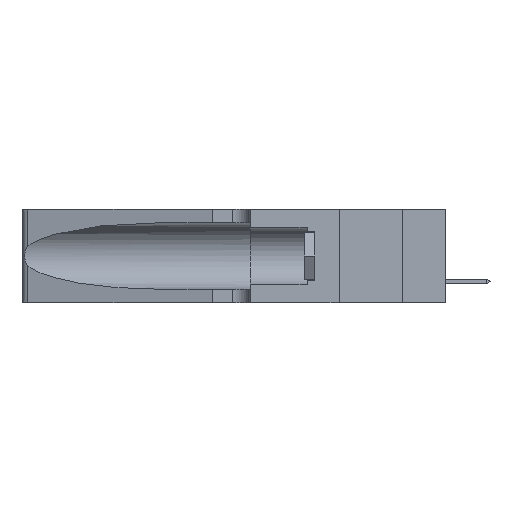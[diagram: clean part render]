
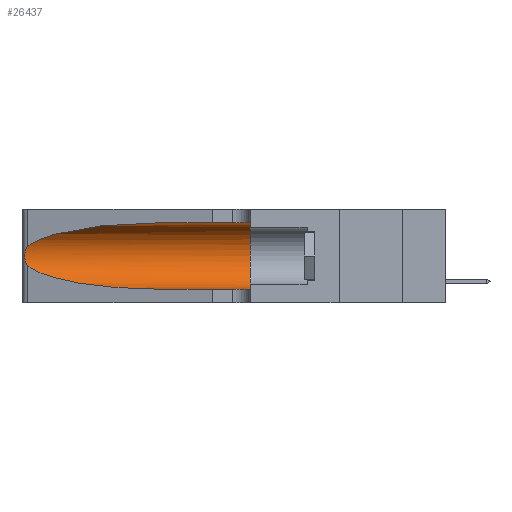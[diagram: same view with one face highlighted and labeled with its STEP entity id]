
A CAD part, left-side view. The second image highlights one B-rep face of the part: STEP entity #26437.
In plain terms, the highlighted cylindrical face has radius 3.308 mm (diameter 6.617 mm), a partial arc.
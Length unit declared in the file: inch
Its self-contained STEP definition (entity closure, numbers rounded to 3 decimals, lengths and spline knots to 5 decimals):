
#262 = CARTESIAN_POINT ( 'NONE',  ( 0.25487, 1.22718, 0.22369 ) ) ;
#280 = AXIS2_PLACEMENT_3D ( 'NONE', #3395, #15954, #1688 ) ;
#473 = CARTESIAN_POINT ( 'NONE',  ( 0.18966, 0.96281, 0.05475 ) ) ;
#739 = ORIENTED_EDGE ( 'NONE', *, *, #21418, .T. ) ;
#1464 = FACE_OUTER_BOUND ( 'NONE', #4771, .T. ) ;
#1688 = DIRECTION ( 'NONE',  ( 0., 0., 1. ) ) ;
#2422 = VECTOR ( 'NONE', #12850, 39.37008 ) ;
#2750 = CARTESIAN_POINT ( 'NONE',  ( 0.1305, 0.72297, 0.05475 ) ) ;
#2774 = CYLINDRICAL_SURFACE ( 'NONE', #20808, 0.13025 ) ;
#3172 = EDGE_CURVE ( 'NONE', #17405, #14031, #8732, .T. ) ;
#3395 = CARTESIAN_POINT ( 'NONE',  ( 0.1305, 0.35, 0.185 ) ) ;
#3426 =( BOUNDED_CURVE ( )  B_SPLINE_CURVE ( 3, ( #11892, #24066, #5710, #11695 ),
 .UNSPECIFIED., .F., .F. ) 
 B_SPLINE_CURVE_WITH_KNOTS ( ( 4, 4 ),
 ( 1.5708, 2.84003 ),
 .UNSPECIFIED. ) 
 CURVE ( )  GEOMETRIC_REPRESENTATION_ITEM ( )  RATIONAL_B_SPLINE_CURVE ( ( 1., 0.87, 0.87, 1. ) ) 
 REPRESENTATION_ITEM ( '' )  );
#4771 = EDGE_LOOP ( 'NONE', ( #6231, #12596, #739, #5840, #10769, #9035 ) ) ;
#5710 = CARTESIAN_POINT ( 'NONE',  ( 0.2373, 1.15595, 0.28018 ) ) ;
#5840 = ORIENTED_EDGE ( 'NONE', *, *, #8519, .T. ) ;
#5871 = CARTESIAN_POINT ( 'NONE',  ( 0.26075, 1.23896, 0.19203 ) ) ;
#6231 = ORIENTED_EDGE ( 'NONE', *, *, #8650, .T. ) ;
#6250 = CARTESIAN_POINT ( 'NONE',  ( 0.1305, 1.61858, 0.185 ) ) ;
#6692 = B_SPLINE_CURVE_WITH_KNOTS ( 'NONE', 3,
 ( #9997, #18161, #20067, #20337, #9913, #26435, #5871, #24551, #7944, #8099, #17982, #26612, #24391, #8023 ),
 .UNSPECIFIED., .F., .F.,
 ( 4, 2, 2, 2, 2, 2, 4 ),
 ( 0., 0.00027, 0.00053, 0.00107, 0.0016, 0.00187, 0.00214 ),
 .UNSPECIFIED. ) ;
#7007 = CARTESIAN_POINT ( 'NONE',  ( 0.25487, 1.22718, 0.14631 ) ) ;
#7218 = CARTESIAN_POINT ( 'NONE',  ( 0.1305, 0.35, 0.31525 ) ) ;
#7944 = CARTESIAN_POINT ( 'NONE',  ( 0.26017, 1.23833, 0.17102 ) ) ;
#8023 = CARTESIAN_POINT ( 'NONE',  ( 0.25487, 1.22718, 0.14631 ) ) ;
#8099 = CARTESIAN_POINT ( 'NONE',  ( 0.25856, 1.23593, 0.16098 ) ) ;
#8519 = EDGE_CURVE ( 'NONE', #26470, #14031, #17799, .T. ) ;
#8650 = EDGE_CURVE ( 'NONE', #16232, #22235, #3426, .T. ) ;
#8732 = CIRCLE ( 'NONE', #280, 0.13025 ) ;
#9035 = ORIENTED_EDGE ( 'NONE', *, *, #17754, .F. ) ;
#9550 = CARTESIAN_POINT ( 'NONE',  ( 0.1305, 0.35, 0.05475 ) ) ;
#9913 = CARTESIAN_POINT ( 'NONE',  ( 0.25854, 1.2359, 0.20912 ) ) ;
#9997 = CARTESIAN_POINT ( 'NONE',  ( 0.25487, 1.22718, 0.22369 ) ) ;
#10358 = CARTESIAN_POINT ( 'NONE',  ( 0.1305, 0.72297, 0.05475 ) ) ;
#10769 = ORIENTED_EDGE ( 'NONE', *, *, #3172, .F. ) ;
#11212 = EDGE_CURVE ( 'NONE', #22235, #25212, #6692, .T. ) ;
#11695 = CARTESIAN_POINT ( 'NONE',  ( 0.25487, 1.22718, 0.22369 ) ) ;
#11892 = CARTESIAN_POINT ( 'NONE',  ( 0.1305, 0.72297, 0.31525 ) ) ;
#12054 = VECTOR ( 'NONE', #23234, 39.37008 ) ;
#12596 = ORIENTED_EDGE ( 'NONE', *, *, #11212, .T. ) ;
#12850 = DIRECTION ( 'NONE',  ( 0., -1., 0. ) ) ;
#13142 = CARTESIAN_POINT ( 'NONE',  ( 0.1305, 1.61858, 0.05475 ) ) ;
#14031 = VERTEX_POINT ( 'NONE', #9550 ) ;
#14220 = CARTESIAN_POINT ( 'NONE',  ( 0.1305, 0.72297, 0.31525 ) ) ;
#14413 = DIRECTION ( 'NONE',  ( 0., -1., 0. ) ) ;
#14416 = CARTESIAN_POINT ( 'NONE',  ( 0.2373, 1.15595, 0.08982 ) ) ;
#15954 = DIRECTION ( 'NONE',  ( 0., 1., 0. ) ) ;
#16232 = VERTEX_POINT ( 'NONE', #14220 ) ;
#16813 = CARTESIAN_POINT ( 'NONE',  ( 0.1305, 1.61858, 0.31525 ) ) ;
#17049 =( BOUNDED_CURVE ( )  B_SPLINE_CURVE ( 3, ( #22644, #14416, #473, #2750 ),
 .UNSPECIFIED., .F., .F. ) 
 B_SPLINE_CURVE_WITH_KNOTS ( ( 4, 4 ),
 ( 3.44316, 4.71239 ),
 .UNSPECIFIED. ) 
 CURVE ( )  GEOMETRIC_REPRESENTATION_ITEM ( )  RATIONAL_B_SPLINE_CURVE ( ( 1., 0.87, 0.87, 1. ) ) 
 REPRESENTATION_ITEM ( '' )  );
#17405 = VERTEX_POINT ( 'NONE', #7218 ) ;
#17754 = EDGE_CURVE ( 'NONE', #16232, #17405, #19443, .T. ) ;
#17799 = LINE ( 'NONE', #13142, #12054 ) ;
#17982 = CARTESIAN_POINT ( 'NONE',  ( 0.25789, 1.23486, 0.15765 ) ) ;
#18161 = CARTESIAN_POINT ( 'NONE',  ( 0.25555, 1.22994, 0.2215 ) ) ;
#19443 = LINE ( 'NONE', #16813, #2422 ) ;
#20067 = CARTESIAN_POINT ( 'NONE',  ( 0.25639, 1.23184, 0.21858 ) ) ;
#20337 = CARTESIAN_POINT ( 'NONE',  ( 0.25787, 1.23484, 0.2124 ) ) ;
#20808 = AXIS2_PLACEMENT_3D ( 'NONE', #6250, #14413, #24833 ) ;
#21418 = EDGE_CURVE ( 'NONE', #25212, #26470, #17049, .T. ) ;
#22235 = VERTEX_POINT ( 'NONE', #262 ) ;
#22644 = CARTESIAN_POINT ( 'NONE',  ( 0.25487, 1.22718, 0.14631 ) ) ;
#23234 = DIRECTION ( 'NONE',  ( 0., -1., 0. ) ) ;
#24066 = CARTESIAN_POINT ( 'NONE',  ( 0.18966, 0.96281, 0.31525 ) ) ;
#24391 = CARTESIAN_POINT ( 'NONE',  ( 0.25555, 1.22993, 0.14849 ) ) ;
#24551 = CARTESIAN_POINT ( 'NONE',  ( 0.26075, 1.23896, 0.178 ) ) ;
#24833 = DIRECTION ( 'NONE',  ( 0., 0., -1. ) ) ;
#25212 = VERTEX_POINT ( 'NONE', #7007 ) ;
#26435 = CARTESIAN_POINT ( 'NONE',  ( 0.26018, 1.23835, 0.19895 ) ) ;
#26437 = ADVANCED_FACE ( 'NONE', ( #1464 ), #2774, .F. ) ;
#26470 = VERTEX_POINT ( 'NONE', #10358 ) ;
#26612 = CARTESIAN_POINT ( 'NONE',  ( 0.25639, 1.23186, 0.15144 ) ) ;
